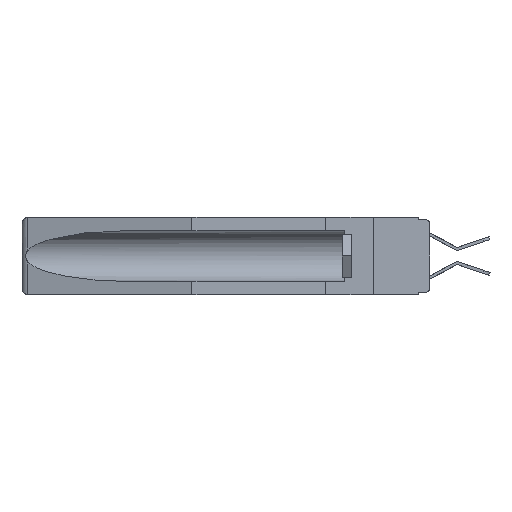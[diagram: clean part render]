
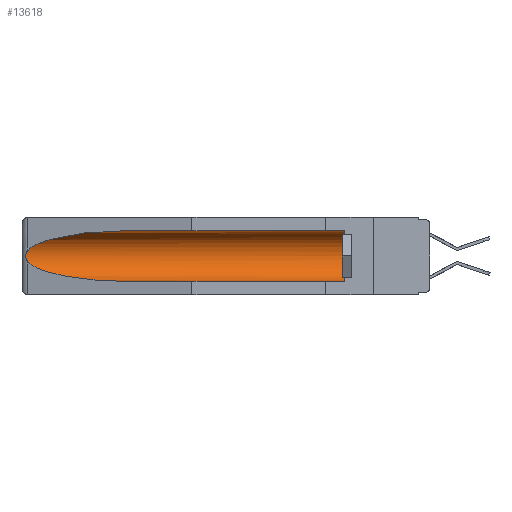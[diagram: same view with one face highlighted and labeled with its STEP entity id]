
A CAD part, left-side view. The second image highlights one B-rep face of the part: STEP entity #13618.
In plain terms, the highlighted cylindrical face has radius 2.857 mm (diameter 5.715 mm), a partial arc.
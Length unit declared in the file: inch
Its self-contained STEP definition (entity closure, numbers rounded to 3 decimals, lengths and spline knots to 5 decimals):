
#21 = CARTESIAN_POINT ( 'NONE',  ( 0.155, 0.126, -0.1715 ) ) ;
#98 = CARTESIAN_POINT ( 'NONE',  ( 0.2673, 1.5327, -0.16383 ) ) ;
#116 = EDGE_CURVE ( 'NONE', #5448, #9837, #7374, .T. ) ;
#236 = VECTOR ( 'NONE', #5057, 39.37008 ) ;
#412 = CARTESIAN_POINT ( 'NONE',  ( 0.155, 0.126, -0.284 ) ) ;
#850 = LINE ( 'NONE', #2476, #236 ) ;
#880 = CARTESIAN_POINT ( 'NONE',  ( 0.26537, 1.52718, -0.19328 ) ) ;
#1401 = DIRECTION ( 'NONE',  ( 0., 1., 0. ) ) ;
#1406 = CARTESIAN_POINT ( 'NONE',  ( 0.26537, 1.52718, -0.14972 ) ) ;
#1455 = ORIENTED_EDGE ( 'NONE', *, *, #116, .T. ) ;
#1555 = CARTESIAN_POINT ( 'NONE',  ( 0.26597, 1.5296, -0.19026 ) ) ;
#1878 = ORIENTED_EDGE ( 'NONE', *, *, #14705, .T. ) ;
#1984 = ORIENTED_EDGE ( 'NONE', *, *, #9611, .T. ) ;
#2125 = CARTESIAN_POINT ( 'NONE',  ( 0.155, 1.07973, -0.059 ) ) ;
#2376 = CARTESIAN_POINT ( 'NONE',  ( 0.155, 1.07973, -0.284 ) ) ;
#2476 = CARTESIAN_POINT ( 'NONE',  ( 0.155, -0.30754, -0.284 ) ) ;
#2750 = CARTESIAN_POINT ( 'NONE',  ( 0.26654, 1.53092, -0.15636 ) ) ;
#2875 = VERTEX_POINT ( 'NONE', #13417 ) ;
#3131 = CARTESIAN_POINT ( 'NONE',  ( 0.155, 1.07973, -0.059 ) ) ;
#3171 = DIRECTION ( 'NONE',  ( 0., 1., 0. ) ) ;
#4179 = ORIENTED_EDGE ( 'NONE', *, *, #13864, .T. ) ;
#5010 =( BOUNDED_CURVE ( )  B_SPLINE_CURVE ( 3, ( #880, #6329, #8955, #2376 ),
 .UNSPECIFIED., .F., .F. ) 
 B_SPLINE_CURVE_WITH_KNOTS ( ( 4, 4 ),
 ( 0.1948, 1.5708 ),
 .UNSPECIFIED. ) 
 CURVE ( )  GEOMETRIC_REPRESENTATION_ITEM ( )  RATIONAL_B_SPLINE_CURVE ( ( 1., 0.848, 0.848, 1. ) ) 
 REPRESENTATION_ITEM ( '' )  );
#5057 = DIRECTION ( 'NONE',  ( 0., 1., 0. ) ) ;
#5295 = AXIS2_PLACEMENT_3D ( 'NONE', #7998, #1401, #15954 ) ;
#5448 = VERTEX_POINT ( 'NONE', #2125 ) ;
#5794 = FACE_OUTER_BOUND ( 'NONE', #7756, .T. ) ;
#6315 = CARTESIAN_POINT ( 'NONE',  ( 0.155, 0.126, -0.059 ) ) ;
#6329 = CARTESIAN_POINT ( 'NONE',  ( 0.25451, 1.48313, -0.24835 ) ) ;
#6559 = DIRECTION ( 'NONE',  ( 0., 0., 1. ) ) ;
#7156 = ORIENTED_EDGE ( 'NONE', *, *, #12344, .T. ) ;
#7374 =( BOUNDED_CURVE ( )  B_SPLINE_CURVE ( 3, ( #3131, #8057, #9412, #1406 ),
 .UNSPECIFIED., .F., .F. ) 
 B_SPLINE_CURVE_WITH_KNOTS ( ( 4, 4 ),
 ( 4.71239, 6.08839 ),
 .UNSPECIFIED. ) 
 CURVE ( )  GEOMETRIC_REPRESENTATION_ITEM ( )  RATIONAL_B_SPLINE_CURVE ( ( 1., 0.848, 0.848, 1. ) ) 
 REPRESENTATION_ITEM ( '' )  );
#7756 = EDGE_LOOP ( 'NONE', ( #1455, #1984, #1878, #13604, #7156, #4179 ) ) ;
#7998 = CARTESIAN_POINT ( 'NONE',  ( 0.155, -0.30754, -0.1715 ) ) ;
#8057 = CARTESIAN_POINT ( 'NONE',  ( 0.21114, 1.30732, -0.059 ) ) ;
#8073 = DIRECTION ( 'NONE',  ( 0., -1., 0. ) ) ;
#8210 = CARTESIAN_POINT ( 'NONE',  ( 0.26537, 1.52718, -0.14972 ) ) ;
#8326 = CARTESIAN_POINT ( 'NONE',  ( 0.2675, 1.53308, -0.17534 ) ) ;
#8665 = CARTESIAN_POINT ( 'NONE',  ( 0.26537, 1.52718, -0.14972 ) ) ;
#8955 = CARTESIAN_POINT ( 'NONE',  ( 0.21114, 1.30732, -0.284 ) ) ;
#9412 = CARTESIAN_POINT ( 'NONE',  ( 0.25451, 1.48313, -0.09465 ) ) ;
#9554 = CARTESIAN_POINT ( 'NONE',  ( 0.2675, 1.53308, -0.16763 ) ) ;
#9611 = EDGE_CURVE ( 'NONE', #9837, #10670, #9956, .T. ) ;
#9837 = VERTEX_POINT ( 'NONE', #8665 ) ;
#9871 = CARTESIAN_POINT ( 'NONE',  ( 0.155, -0.30754, -0.059 ) ) ;
#9956 = B_SPLINE_CURVE_WITH_KNOTS ( 'NONE', 3,
 ( #8210, #12238, #2750, #98, #9554, #8326, #12133, #10906, #1555, #14856 ),
 .UNSPECIFIED., .F., .F.,
 ( 4, 2, 2, 2, 4 ),
 ( 0., 0.00029, 0.00058, 0.00087, 0.00117 ),
 .UNSPECIFIED. ) ;
#10670 = VERTEX_POINT ( 'NONE', #13168 ) ;
#10906 = CARTESIAN_POINT ( 'NONE',  ( 0.26655, 1.53094, -0.18657 ) ) ;
#11173 = EDGE_CURVE ( 'NONE', #15082, #2875, #850, .T. ) ;
#12012 = AXIS2_PLACEMENT_3D ( 'NONE', #21, #8073, #6559 ) ;
#12042 = LINE ( 'NONE', #9871, #16292 ) ;
#12133 = CARTESIAN_POINT ( 'NONE',  ( 0.2673, 1.53269, -0.17917 ) ) ;
#12238 = CARTESIAN_POINT ( 'NONE',  ( 0.26597, 1.52961, -0.15275 ) ) ;
#12344 = EDGE_CURVE ( 'NONE', #15082, #13368, #13388, .T. ) ;
#13168 = CARTESIAN_POINT ( 'NONE',  ( 0.26537, 1.52718, -0.19328 ) ) ;
#13368 = VERTEX_POINT ( 'NONE', #6315 ) ;
#13388 = CIRCLE ( 'NONE', #12012, 0.1125 ) ;
#13417 = CARTESIAN_POINT ( 'NONE',  ( 0.155, 1.07973, -0.284 ) ) ;
#13604 = ORIENTED_EDGE ( 'NONE', *, *, #11173, .F. ) ;
#13618 = ADVANCED_FACE ( 'NONE', ( #5794 ), #16929, .F. ) ;
#13864 = EDGE_CURVE ( 'NONE', #13368, #5448, #12042, .T. ) ;
#14705 = EDGE_CURVE ( 'NONE', #10670, #2875, #5010, .T. ) ;
#14856 = CARTESIAN_POINT ( 'NONE',  ( 0.26537, 1.52718, -0.19328 ) ) ;
#15082 = VERTEX_POINT ( 'NONE', #412 ) ;
#15954 = DIRECTION ( 'NONE',  ( 0., 0., 1. ) ) ;
#16292 = VECTOR ( 'NONE', #3171, 39.37008 ) ;
#16929 = CYLINDRICAL_SURFACE ( 'NONE', #5295, 0.1125 ) ;
